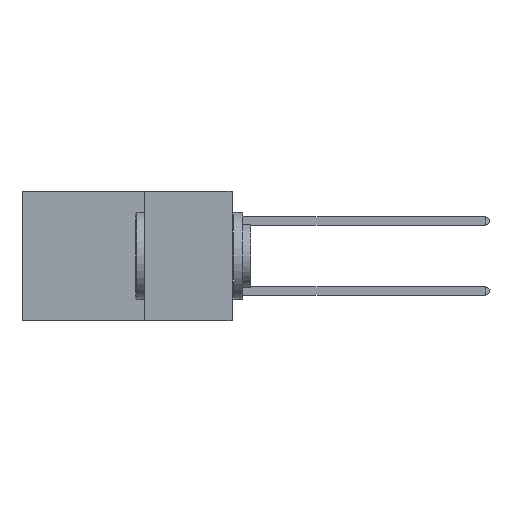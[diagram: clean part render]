
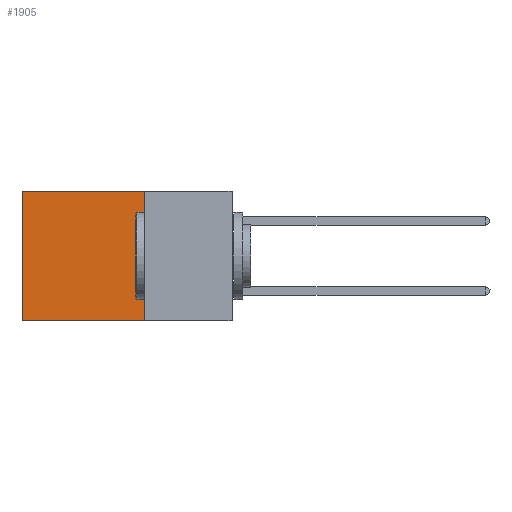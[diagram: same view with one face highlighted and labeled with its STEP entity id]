
A CAD part, left-side view. The second image highlights one B-rep face of the part: STEP entity #1905.
In plain terms, the highlighted planar face has unit normal (-1, 0, 0).
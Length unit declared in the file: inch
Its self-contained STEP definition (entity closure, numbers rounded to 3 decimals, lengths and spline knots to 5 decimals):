
#511 = LINE ( 'NONE', #11448, #14874 ) ;
#606 = PLANE ( 'NONE',  #2081 ) ;
#1464 = CARTESIAN_POINT ( 'NONE',  ( 0.2875, 0.25, -0.37 ) ) ;
#1567 = VERTEX_POINT ( 'NONE', #11428 ) ;
#1905 = ADVANCED_FACE ( 'NONE', ( #7360 ), #606, .F. ) ;
#2081 = AXIS2_PLACEMENT_3D ( 'NONE', #11340, #8813, #6393 ) ;
#2355 = VERTEX_POINT ( 'NONE', #9552 ) ;
#2493 = ORIENTED_EDGE ( 'NONE', *, *, #15368, .F. ) ;
#3500 = CARTESIAN_POINT ( 'NONE',  ( 0.2875, 0.25, 0. ) ) ;
#3555 = ORIENTED_EDGE ( 'NONE', *, *, #7277, .F. ) ;
#5420 = CARTESIAN_POINT ( 'NONE',  ( 0.2875, 0.25, -0.37 ) ) ;
#5620 = EDGE_CURVE ( 'NONE', #14608, #2355, #14061, .T. ) ;
#5672 = DIRECTION ( 'NONE',  ( 0., 1., 0. ) ) ;
#5685 = ORIENTED_EDGE ( 'NONE', *, *, #11738, .T. ) ;
#6350 = VECTOR ( 'NONE', #8892, 39.37008 ) ;
#6393 = DIRECTION ( 'NONE',  ( 0., 0., -1. ) ) ;
#6511 = CARTESIAN_POINT ( 'NONE',  ( 0.2875, 0.25, 0. ) ) ;
#6682 = EDGE_LOOP ( 'NONE', ( #5685, #2493, #3555, #9896 ) ) ;
#6750 = DIRECTION ( 'NONE',  ( 0., 0., -1. ) ) ;
#6780 = VECTOR ( 'NONE', #7112, 39.37008 ) ;
#6814 = VECTOR ( 'NONE', #5672, 39.37008 ) ;
#7112 = DIRECTION ( 'NONE',  ( 0., 1., 0. ) ) ;
#7277 = EDGE_CURVE ( 'NONE', #14608, #11974, #12702, .T. ) ;
#7360 = FACE_OUTER_BOUND ( 'NONE', #6682, .T. ) ;
#8307 = LINE ( 'NONE', #5420, #6814 ) ;
#8712 = CARTESIAN_POINT ( 'NONE',  ( 0.2875, 0.25, 0. ) ) ;
#8813 = DIRECTION ( 'NONE',  ( 1., 0., 0. ) ) ;
#8892 = DIRECTION ( 'NONE',  ( 0., 0., -1. ) ) ;
#9552 = CARTESIAN_POINT ( 'NONE',  ( 0.2875, 0.6, 0. ) ) ;
#9896 = ORIENTED_EDGE ( 'NONE', *, *, #5620, .T. ) ;
#11340 = CARTESIAN_POINT ( 'NONE',  ( 0.2875, 0.25, 0. ) ) ;
#11428 = CARTESIAN_POINT ( 'NONE',  ( 0.2875, 0.6, -0.37 ) ) ;
#11448 = CARTESIAN_POINT ( 'NONE',  ( 0.2875, 0.6, 0. ) ) ;
#11738 = EDGE_CURVE ( 'NONE', #2355, #1567, #511, .T. ) ;
#11974 = VERTEX_POINT ( 'NONE', #1464 ) ;
#12702 = LINE ( 'NONE', #6511, #6350 ) ;
#14061 = LINE ( 'NONE', #3500, #6780 ) ;
#14608 = VERTEX_POINT ( 'NONE', #8712 ) ;
#14874 = VECTOR ( 'NONE', #6750, 39.37008 ) ;
#15368 = EDGE_CURVE ( 'NONE', #11974, #1567, #8307, .T. ) ;
